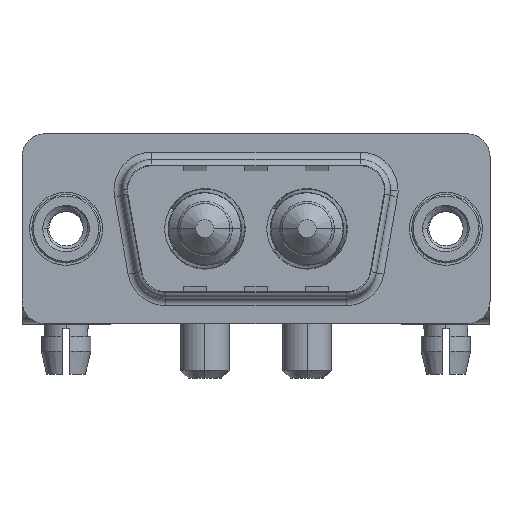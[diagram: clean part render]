
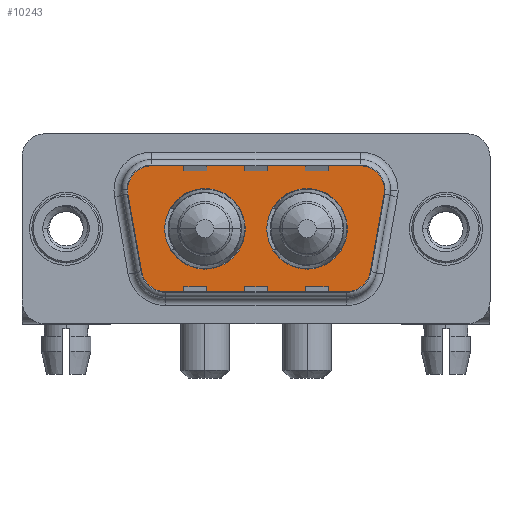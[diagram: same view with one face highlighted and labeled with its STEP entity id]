
A CAD part, top view. The second image highlights one B-rep face of the part: STEP entity #10243.
In plain terms, the highlighted planar face has unit normal (0, 0, 1).
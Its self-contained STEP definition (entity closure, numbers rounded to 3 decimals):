
#166 = CIRCLE ( 'NONE', #8924, 2.65 ) ;
#261 = CARTESIAN_POINT ( 'NONE',  ( 21.564, 2.9, 0. ) ) ;
#403 = ORIENTED_EDGE ( 'NONE', *, *, #3657, .T. ) ;
#480 = CIRCLE ( 'NONE', #13885, 2.65 ) ;
#708 = VERTEX_POINT ( 'NONE', #13144 ) ;
#808 = ORIENTED_EDGE ( 'NONE', *, *, #14635, .T. ) ;
#811 = DIRECTION ( 'NONE',  ( 0., 0., 1. ) ) ;
#1044 = CIRCLE ( 'NONE', #9553, 2. ) ;
#1155 = VECTOR ( 'NONE', #3745, 1000. ) ;
#1172 = CARTESIAN_POINT ( 'NONE',  ( 11.79, 0., 0. ) ) ;
#1292 = LINE ( 'NONE', #15106, #10906 ) ;
#1442 = CARTESIAN_POINT ( 'NONE',  ( 19.564, 2.9, 0. ) ) ;
#1457 = DIRECTION ( 'NONE',  ( 1., 0., 0. ) ) ;
#1495 = ORIENTED_EDGE ( 'NONE', *, *, #12450, .T. ) ;
#1535 = CARTESIAN_POINT ( 'NONE',  ( 19.564, 2.9, 0. ) ) ;
#1560 = DIRECTION ( 'NONE',  ( 1., 0., 0. ) ) ;
#1642 = CARTESIAN_POINT ( 'NONE',  ( 13.21, 0., 0. ) ) ;
#1963 = EDGE_LOOP ( 'NONE', ( #13904, #7054 ) ) ;
#2023 = AXIS2_PLACEMENT_3D ( 'NONE', #1535, #9759, #13294 ) ;
#2386 = VERTEX_POINT ( 'NONE', #3248 ) ;
#2414 = AXIS2_PLACEMENT_3D ( 'NONE', #1442, #2736, #7368 ) ;
#2498 = DIRECTION ( 'NONE',  ( 0., 0., 1. ) ) ;
#2513 = DIRECTION ( 'NONE',  ( -1., 0., 0. ) ) ;
#2653 = CIRCLE ( 'NONE', #5571, 2.65 ) ;
#2734 = AXIS2_PLACEMENT_3D ( 'NONE', #6411, #7626, #12310 ) ;
#2736 = DIRECTION ( 'NONE',  ( 0., 0., 1. ) ) ;
#2785 = LINE ( 'NONE', #7338, #4008 ) ;
#2925 = VECTOR ( 'NONE', #3338, 1000. ) ;
#3033 = CARTESIAN_POINT ( 'NONE',  ( 5.436, 4.9, 0. ) ) ;
#3140 = EDGE_CURVE ( 'NONE', #10094, #11891, #166, .T. ) ;
#3217 = ORIENTED_EDGE ( 'NONE', *, *, #14089, .T. ) ;
#3248 = CARTESIAN_POINT ( 'NONE',  ( 19.564, 4.9, 0. ) ) ;
#3338 = DIRECTION ( 'NONE',  ( 0.174, 0.985, 0. ) ) ;
#3482 = CIRCLE ( 'NONE', #2023, 2. ) ;
#3502 = DIRECTION ( 'NONE',  ( -1., 0., 0. ) ) ;
#3525 = EDGE_CURVE ( 'NONE', #2386, #9250, #1292, .T. ) ;
#3657 = EDGE_CURVE ( 'NONE', #708, #5923, #8672, .T. ) ;
#3745 = DIRECTION ( 'NONE',  ( 0.174, -0.985, 0. ) ) ;
#3907 = ORIENTED_EDGE ( 'NONE', *, *, #3525, .T. ) ;
#3941 = EDGE_LOOP ( 'NONE', ( #8215, #11028 ) ) ;
#3948 = CARTESIAN_POINT ( 'NONE',  ( 18.541, -4.9, 0. ) ) ;
#3977 = ORIENTED_EDGE ( 'NONE', *, *, #7508, .T. ) ;
#4008 = VECTOR ( 'NONE', #1560, 1000. ) ;
#4259 = CARTESIAN_POINT ( 'NONE',  ( 21.534, 2.553, 0. ) ) ;
#4802 = AXIS2_PLACEMENT_3D ( 'NONE', #11999, #9692, #5967 ) ;
#4822 = EDGE_CURVE ( 'NONE', #6457, #11978, #2653, .T. ) ;
#4990 = CIRCLE ( 'NONE', #6146, 2. ) ;
#5571 = AXIS2_PLACEMENT_3D ( 'NONE', #12526, #6709, #7995 ) ;
#5923 = VERTEX_POINT ( 'NONE', #11623 ) ;
#5967 = DIRECTION ( 'NONE',  ( 1., 0., 0. ) ) ;
#6037 = DIRECTION ( 'NONE',  ( 1., 0., 0. ) ) ;
#6122 = EDGE_CURVE ( 'NONE', #11891, #10094, #480, .T. ) ;
#6146 = AXIS2_PLACEMENT_3D ( 'NONE', #14111, #2498, #3502 ) ;
#6195 = EDGE_CURVE ( 'NONE', #11530, #8278, #14858, .T. ) ;
#6411 = CARTESIAN_POINT ( 'NONE',  ( 18.541, -2.9, 0. ) ) ;
#6457 = VERTEX_POINT ( 'NONE', #1172 ) ;
#6709 = DIRECTION ( 'NONE',  ( 0., 0., 1. ) ) ;
#7054 = ORIENTED_EDGE ( 'NONE', *, *, #13828, .F. ) ;
#7198 = CARTESIAN_POINT ( 'NONE',  ( 6.49, 0., 0. ) ) ;
#7251 = CARTESIAN_POINT ( 'NONE',  ( 18.51, 0., 0. ) ) ;
#7303 = CARTESIAN_POINT ( 'NONE',  ( 3.466, 2.553, 0. ) ) ;
#7338 = CARTESIAN_POINT ( 'NONE',  ( 6.459, -4.9, 0. ) ) ;
#7368 = DIRECTION ( 'NONE',  ( -1., 0., 0. ) ) ;
#7391 = DIRECTION ( 'NONE',  ( 1., 0., 0. ) ) ;
#7508 = EDGE_CURVE ( 'NONE', #8278, #8825, #11688, .T. ) ;
#7626 = DIRECTION ( 'NONE',  ( 0., 0., 1. ) ) ;
#7883 = AXIS2_PLACEMENT_3D ( 'NONE', #14775, #811, #12263 ) ;
#7947 = ORIENTED_EDGE ( 'NONE', *, *, #12478, .T. ) ;
#7995 = DIRECTION ( 'NONE',  ( 1., 0., 0. ) ) ;
#8215 = ORIENTED_EDGE ( 'NONE', *, *, #3140, .F. ) ;
#8278 = VERTEX_POINT ( 'NONE', #10417 ) ;
#8383 = CARTESIAN_POINT ( 'NONE',  ( 15.86, 0., 0. ) ) ;
#8391 = DIRECTION ( 'NONE',  ( 0., 0., 1. ) ) ;
#8648 = VERTEX_POINT ( 'NONE', #10399 ) ;
#8672 = LINE ( 'NONE', #7303, #1155 ) ;
#8770 = FACE_BOUND ( 'NONE', #1963, .T. ) ;
#8825 = VERTEX_POINT ( 'NONE', #261 ) ;
#8919 = PLANE ( 'NONE',  #2734 ) ;
#8924 = AXIS2_PLACEMENT_3D ( 'NONE', #13296, #8391, #7391 ) ;
#8997 = FACE_OUTER_BOUND ( 'NONE', #14893, .T. ) ;
#9106 = CIRCLE ( 'NONE', #7883, 2.65 ) ;
#9250 = VERTEX_POINT ( 'NONE', #3033 ) ;
#9553 = AXIS2_PLACEMENT_3D ( 'NONE', #12993, #10324, #6037 ) ;
#9692 = DIRECTION ( 'NONE',  ( 0., 0., 1. ) ) ;
#9759 = DIRECTION ( 'NONE',  ( 0., 0., 1. ) ) ;
#9868 = ORIENTED_EDGE ( 'NONE', *, *, #6195, .T. ) ;
#10094 = VERTEX_POINT ( 'NONE', #7251 ) ;
#10110 = CARTESIAN_POINT ( 'NONE',  ( 20.511, -3.247, 0. ) ) ;
#10148 = FACE_BOUND ( 'NONE', #3941, .T. ) ;
#10243 = ADVANCED_FACE ( 'NONE', ( #10148, #8770, #8997 ), #8919, .T. ) ;
#10324 = DIRECTION ( 'NONE',  ( 0., 0., 1. ) ) ;
#10399 = CARTESIAN_POINT ( 'NONE',  ( 6.459, -4.9, 0. ) ) ;
#10417 = CARTESIAN_POINT ( 'NONE',  ( 21.534, 2.553, 0. ) ) ;
#10906 = VECTOR ( 'NONE', #2513, 1000. ) ;
#11028 = ORIENTED_EDGE ( 'NONE', *, *, #6122, .F. ) ;
#11530 = VERTEX_POINT ( 'NONE', #10110 ) ;
#11623 = CARTESIAN_POINT ( 'NONE',  ( 4.489, -3.247, 0. ) ) ;
#11688 = CIRCLE ( 'NONE', #2414, 2. ) ;
#11891 = VERTEX_POINT ( 'NONE', #1642 ) ;
#11978 = VERTEX_POINT ( 'NONE', #7198 ) ;
#11999 = CARTESIAN_POINT ( 'NONE',  ( 5.436, 2.9, 0. ) ) ;
#12263 = DIRECTION ( 'NONE',  ( 1., 0., 0. ) ) ;
#12288 = EDGE_CURVE ( 'NONE', #13085, #11530, #1044, .T. ) ;
#12310 = DIRECTION ( 'NONE',  ( 1., 0., 0. ) ) ;
#12450 = EDGE_CURVE ( 'NONE', #8825, #2386, #3482, .T. ) ;
#12478 = EDGE_CURVE ( 'NONE', #5923, #8648, #4990, .T. ) ;
#12526 = CARTESIAN_POINT ( 'NONE',  ( 9.14, 0., 0. ) ) ;
#12832 = CIRCLE ( 'NONE', #4802, 2. ) ;
#12993 = CARTESIAN_POINT ( 'NONE',  ( 18.541, -2.9, 0. ) ) ;
#13065 = DIRECTION ( 'NONE',  ( 0., 0., 1. ) ) ;
#13085 = VERTEX_POINT ( 'NONE', #3948 ) ;
#13144 = CARTESIAN_POINT ( 'NONE',  ( 3.466, 2.553, 0. ) ) ;
#13294 = DIRECTION ( 'NONE',  ( -1., 0., 0. ) ) ;
#13296 = CARTESIAN_POINT ( 'NONE',  ( 15.86, 0., 0. ) ) ;
#13475 = ORIENTED_EDGE ( 'NONE', *, *, #12288, .T. ) ;
#13828 = EDGE_CURVE ( 'NONE', #11978, #6457, #9106, .T. ) ;
#13885 = AXIS2_PLACEMENT_3D ( 'NONE', #8383, #13065, #1457 ) ;
#13904 = ORIENTED_EDGE ( 'NONE', *, *, #4822, .F. ) ;
#14089 = EDGE_CURVE ( 'NONE', #8648, #13085, #2785, .T. ) ;
#14111 = CARTESIAN_POINT ( 'NONE',  ( 6.459, -2.9, 0. ) ) ;
#14635 = EDGE_CURVE ( 'NONE', #9250, #708, #12832, .T. ) ;
#14775 = CARTESIAN_POINT ( 'NONE',  ( 9.14, 0., 0. ) ) ;
#14858 = LINE ( 'NONE', #4259, #2925 ) ;
#14893 = EDGE_LOOP ( 'NONE', ( #13475, #9868, #3977, #1495, #3907, #808, #403, #7947, #3217 ) ) ;
#15106 = CARTESIAN_POINT ( 'NONE',  ( 5.436, 4.9, 0. ) ) ;
